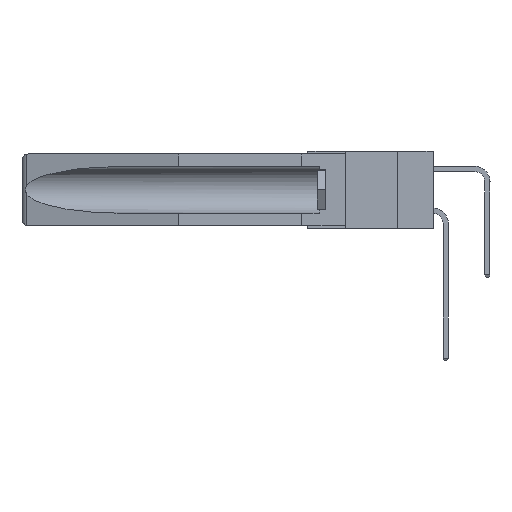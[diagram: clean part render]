
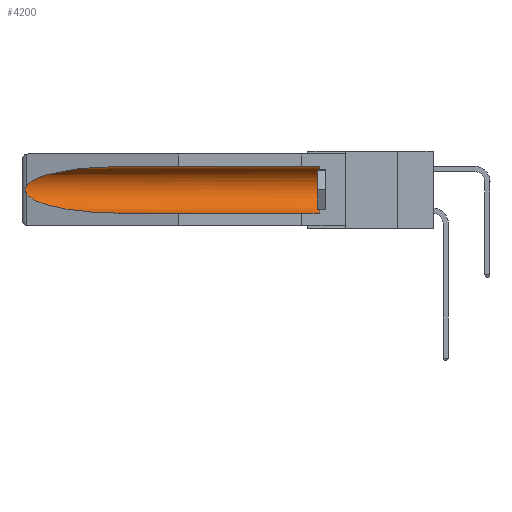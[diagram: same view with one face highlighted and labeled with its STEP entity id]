
A CAD part, left-side view. The second image highlights one B-rep face of the part: STEP entity #4200.
In plain terms, the highlighted cylindrical face has radius 2.857 mm (diameter 5.715 mm), a partial arc.
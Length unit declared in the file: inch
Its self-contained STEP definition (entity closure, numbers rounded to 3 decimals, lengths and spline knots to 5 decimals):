
#100 = CARTESIAN_POINT ( 'NONE',  ( 0.2673, 1.5327, -0.16383 ) ) ;
#266 =( BOUNDED_CURVE ( )  B_SPLINE_CURVE ( 3, ( #15418, #6897, #12355, #23557 ),
 .UNSPECIFIED., .F., .F. ) 
 B_SPLINE_CURVE_WITH_KNOTS ( ( 4, 4 ),
 ( 0.1948, 1.5708 ),
 .UNSPECIFIED. ) 
 CURVE ( )  GEOMETRIC_REPRESENTATION_ITEM ( )  RATIONAL_B_SPLINE_CURVE ( ( 1., 0.848, 0.848, 1. ) ) 
 REPRESENTATION_ITEM ( '' )  );
#363 = ORIENTED_EDGE ( 'NONE', *, *, #11381, .F. ) ;
#2456 = CARTESIAN_POINT ( 'NONE',  ( 0.2675, 1.53308, -0.16763 ) ) ;
#2654 = VERTEX_POINT ( 'NONE', #30362 ) ;
#2694 = CARTESIAN_POINT ( 'NONE',  ( 0.26537, 1.52718, -0.14972 ) ) ;
#3238 = CARTESIAN_POINT ( 'NONE',  ( 0.155, 1.07973, -0.284 ) ) ;
#3314 = DIRECTION ( 'NONE',  ( 0., -1., 0. ) ) ;
#3654 = EDGE_CURVE ( 'NONE', #28016, #9642, #14469, .T. ) ;
#3698 = CIRCLE ( 'NONE', #30340, 0.1125 ) ;
#4200 = ADVANCED_FACE ( 'NONE', ( #7633 ), #34689, .F. ) ;
#5085 = CARTESIAN_POINT ( 'NONE',  ( 0.26654, 1.53092, -0.15636 ) ) ;
#5942 = VERTEX_POINT ( 'NONE', #6813 ) ;
#6813 = CARTESIAN_POINT ( 'NONE',  ( 0.26537, 1.52718, -0.14972 ) ) ;
#6897 = CARTESIAN_POINT ( 'NONE',  ( 0.25451, 1.48313, -0.24835 ) ) ;
#7633 = FACE_OUTER_BOUND ( 'NONE', #21132, .T. ) ;
#7822 = CARTESIAN_POINT ( 'NONE',  ( 0.2673, 1.53269, -0.17917 ) ) ;
#8189 = CARTESIAN_POINT ( 'NONE',  ( 0.155, -0.30754, -0.284 ) ) ;
#8224 = CARTESIAN_POINT ( 'NONE',  ( 0.155, 0.126, -0.059 ) ) ;
#9289 = DIRECTION ( 'NONE',  ( 0., 0., 1. ) ) ;
#9535 = EDGE_CURVE ( 'NONE', #2654, #28016, #3698, .T. ) ;
#9642 = VERTEX_POINT ( 'NONE', #25930 ) ;
#9925 = EDGE_CURVE ( 'NONE', #5942, #12658, #28051, .T. ) ;
#9962 = CARTESIAN_POINT ( 'NONE',  ( 0.155, -0.30754, -0.1715 ) ) ;
#10327 = DIRECTION ( 'NONE',  ( 0., 0., 1. ) ) ;
#10855 = LINE ( 'NONE', #8189, #34928 ) ;
#11381 = EDGE_CURVE ( 'NONE', #2654, #26076, #10855, .T. ) ;
#12020 = ORIENTED_EDGE ( 'NONE', *, *, #9925, .T. ) ;
#12355 = CARTESIAN_POINT ( 'NONE',  ( 0.21114, 1.30732, -0.284 ) ) ;
#12658 = VERTEX_POINT ( 'NONE', #22268 ) ;
#13177 = ORIENTED_EDGE ( 'NONE', *, *, #9535, .T. ) ;
#14469 = LINE ( 'NONE', #23585, #27996 ) ;
#15418 = CARTESIAN_POINT ( 'NONE',  ( 0.26537, 1.52718, -0.19328 ) ) ;
#15628 = ORIENTED_EDGE ( 'NONE', *, *, #26872, .T. ) ;
#15998 = CARTESIAN_POINT ( 'NONE',  ( 0.26655, 1.53094, -0.18657 ) ) ;
#16355 = CARTESIAN_POINT ( 'NONE',  ( 0.26597, 1.52961, -0.15275 ) ) ;
#16362 = DIRECTION ( 'NONE',  ( 0., 1., 0. ) ) ;
#16589 =( BOUNDED_CURVE ( )  B_SPLINE_CURVE ( 3, ( #34882, #27012, #18953, #22245 ),
 .UNSPECIFIED., .F., .F. ) 
 B_SPLINE_CURVE_WITH_KNOTS ( ( 4, 4 ),
 ( 4.71239, 6.08839 ),
 .UNSPECIFIED. ) 
 CURVE ( )  GEOMETRIC_REPRESENTATION_ITEM ( )  RATIONAL_B_SPLINE_CURVE ( ( 1., 0.848, 0.848, 1. ) ) 
 REPRESENTATION_ITEM ( '' )  );
#18123 = DIRECTION ( 'NONE',  ( 0., 1., 0. ) ) ;
#18953 = CARTESIAN_POINT ( 'NONE',  ( 0.25451, 1.48313, -0.09465 ) ) ;
#21132 = EDGE_LOOP ( 'NONE', ( #29350, #12020, #15628, #363, #13177, #31620 ) ) ;
#22245 = CARTESIAN_POINT ( 'NONE',  ( 0.26537, 1.52718, -0.14972 ) ) ;
#22268 = CARTESIAN_POINT ( 'NONE',  ( 0.26537, 1.52718, -0.19328 ) ) ;
#22738 = CARTESIAN_POINT ( 'NONE',  ( 0.155, 0.126, -0.1715 ) ) ;
#23557 = CARTESIAN_POINT ( 'NONE',  ( 0.155, 1.07973, -0.284 ) ) ;
#23585 = CARTESIAN_POINT ( 'NONE',  ( 0.155, -0.30754, -0.059 ) ) ;
#23702 = DIRECTION ( 'NONE',  ( 0., 1., 0. ) ) ;
#24014 = CARTESIAN_POINT ( 'NONE',  ( 0.2675, 1.53308, -0.17534 ) ) ;
#24139 = CARTESIAN_POINT ( 'NONE',  ( 0.26597, 1.5296, -0.19026 ) ) ;
#25930 = CARTESIAN_POINT ( 'NONE',  ( 0.155, 1.07973, -0.059 ) ) ;
#26076 = VERTEX_POINT ( 'NONE', #3238 ) ;
#26872 = EDGE_CURVE ( 'NONE', #12658, #26076, #266, .T. ) ;
#26882 = CARTESIAN_POINT ( 'NONE',  ( 0.26537, 1.52718, -0.19328 ) ) ;
#27012 = CARTESIAN_POINT ( 'NONE',  ( 0.21114, 1.30732, -0.059 ) ) ;
#27996 = VECTOR ( 'NONE', #23702, 39.37008 ) ;
#28016 = VERTEX_POINT ( 'NONE', #8224 ) ;
#28051 = B_SPLINE_CURVE_WITH_KNOTS ( 'NONE', 3,
 ( #2694, #16355, #5085, #100, #2456, #24014, #7822, #15998, #24139, #26882 ),
 .UNSPECIFIED., .F., .F.,
 ( 4, 2, 2, 2, 4 ),
 ( 0., 0.00029, 0.00058, 0.00087, 0.00117 ),
 .UNSPECIFIED. ) ;
#28258 = EDGE_CURVE ( 'NONE', #9642, #5942, #16589, .T. ) ;
#28439 = AXIS2_PLACEMENT_3D ( 'NONE', #9962, #18123, #10327 ) ;
#29350 = ORIENTED_EDGE ( 'NONE', *, *, #28258, .T. ) ;
#30340 = AXIS2_PLACEMENT_3D ( 'NONE', #22738, #3314, #9289 ) ;
#30362 = CARTESIAN_POINT ( 'NONE',  ( 0.155, 0.126, -0.284 ) ) ;
#31620 = ORIENTED_EDGE ( 'NONE', *, *, #3654, .T. ) ;
#34689 = CYLINDRICAL_SURFACE ( 'NONE', #28439, 0.1125 ) ;
#34882 = CARTESIAN_POINT ( 'NONE',  ( 0.155, 1.07973, -0.059 ) ) ;
#34928 = VECTOR ( 'NONE', #16362, 39.37008 ) ;
